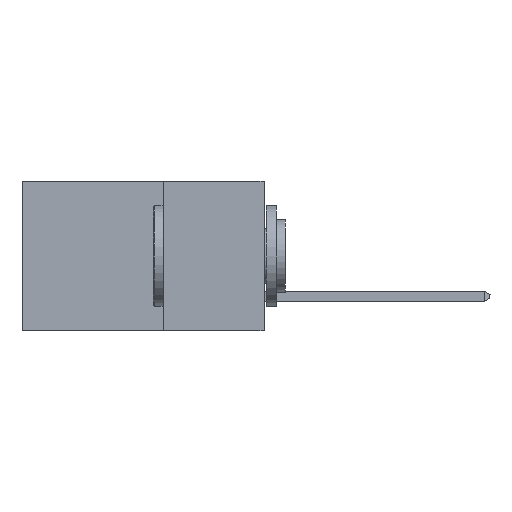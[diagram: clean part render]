
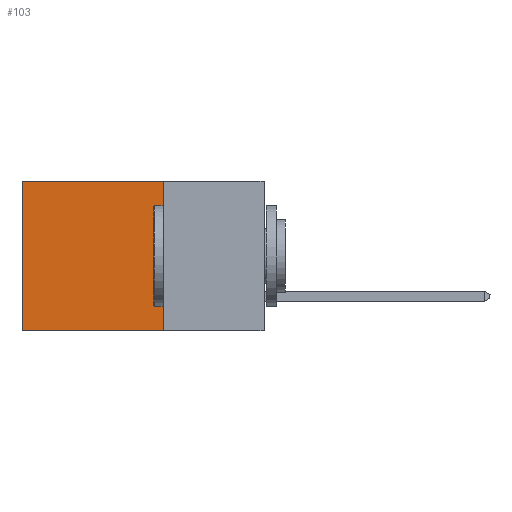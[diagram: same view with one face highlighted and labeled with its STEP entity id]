
A CAD part, left-side view. The second image highlights one B-rep face of the part: STEP entity #103.
In plain terms, the highlighted planar face has unit normal (-1, 0, 0).
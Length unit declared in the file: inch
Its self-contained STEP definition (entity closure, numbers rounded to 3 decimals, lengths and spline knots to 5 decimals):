
#103 = ADVANCED_FACE ( 'NONE', ( #12301 ), #794, .F. ) ;
#789 = VERTEX_POINT ( 'NONE', #9100 ) ;
#794 = PLANE ( 'NONE',  #19714 ) ;
#1985 = VERTEX_POINT ( 'NONE', #5261 ) ;
#2511 = CARTESIAN_POINT ( 'NONE',  ( 0.2615, 0.25, 0. ) ) ;
#2650 = LINE ( 'NONE', #16299, #21058 ) ;
#2722 = DIRECTION ( 'NONE',  ( 0., 1., 0. ) ) ;
#3449 = ORIENTED_EDGE ( 'NONE', *, *, #8867, .F. ) ;
#4433 = EDGE_CURVE ( 'NONE', #22158, #1985, #19539, .T. ) ;
#5261 = CARTESIAN_POINT ( 'NONE',  ( 0.2615, 0.6, 0. ) ) ;
#5300 = EDGE_CURVE ( 'NONE', #22158, #789, #24454, .T. ) ;
#6779 = CARTESIAN_POINT ( 'NONE',  ( 0.2615, 0.25, -0.37 ) ) ;
#7305 = VECTOR ( 'NONE', #2722, 39.37008 ) ;
#8494 = CARTESIAN_POINT ( 'NONE',  ( 0.2615, 0.25, -0.37 ) ) ;
#8867 = EDGE_CURVE ( 'NONE', #789, #15211, #18240, .T. ) ;
#9100 = CARTESIAN_POINT ( 'NONE',  ( 0.2615, 0.25, -0.37 ) ) ;
#10494 = ORIENTED_EDGE ( 'NONE', *, *, #4433, .T. ) ;
#11815 = DIRECTION ( 'NONE',  ( 1., 0., 0. ) ) ;
#12101 = EDGE_LOOP ( 'NONE', ( #18782, #3449, #14468, #10494 ) ) ;
#12185 = VECTOR ( 'NONE', #18279, 39.37008 ) ;
#12301 = FACE_OUTER_BOUND ( 'NONE', #12101, .T. ) ;
#12348 = CARTESIAN_POINT ( 'NONE',  ( 0.2615, 0.6, -0.37 ) ) ;
#12447 = CARTESIAN_POINT ( 'NONE',  ( 0.2615, 0.25, -0.37 ) ) ;
#12766 = DIRECTION ( 'NONE',  ( 0., 0., -1. ) ) ;
#13501 = EDGE_CURVE ( 'NONE', #1985, #15211, #2650, .T. ) ;
#14070 = DIRECTION ( 'NONE',  ( 0., 0., -1. ) ) ;
#14468 = ORIENTED_EDGE ( 'NONE', *, *, #5300, .F. ) ;
#15211 = VERTEX_POINT ( 'NONE', #12348 ) ;
#16299 = CARTESIAN_POINT ( 'NONE',  ( 0.2615, 0.6, -0.37 ) ) ;
#18240 = LINE ( 'NONE', #12447, #22313 ) ;
#18279 = DIRECTION ( 'NONE',  ( 0., 0., -1. ) ) ;
#18782 = ORIENTED_EDGE ( 'NONE', *, *, #13501, .T. ) ;
#19539 = LINE ( 'NONE', #19899, #7305 ) ;
#19714 = AXIS2_PLACEMENT_3D ( 'NONE', #8494, #11815, #14070 ) ;
#19899 = CARTESIAN_POINT ( 'NONE',  ( 0.2615, 0.25, 0. ) ) ;
#21058 = VECTOR ( 'NONE', #12766, 39.37008 ) ;
#22158 = VERTEX_POINT ( 'NONE', #2511 ) ;
#22313 = VECTOR ( 'NONE', #22407, 39.37008 ) ;
#22407 = DIRECTION ( 'NONE',  ( 0., 1., 0. ) ) ;
#24454 = LINE ( 'NONE', #6779, #12185 ) ;
